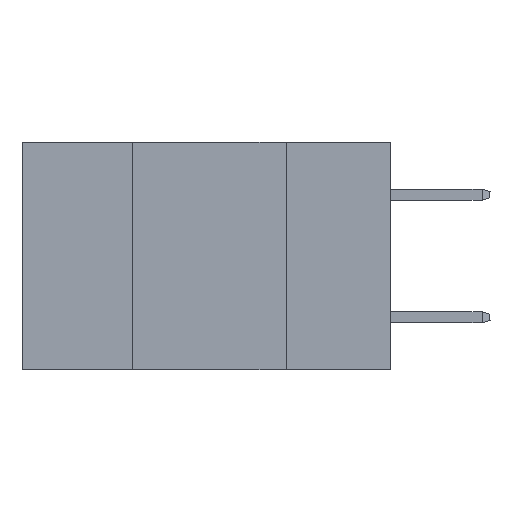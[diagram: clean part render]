
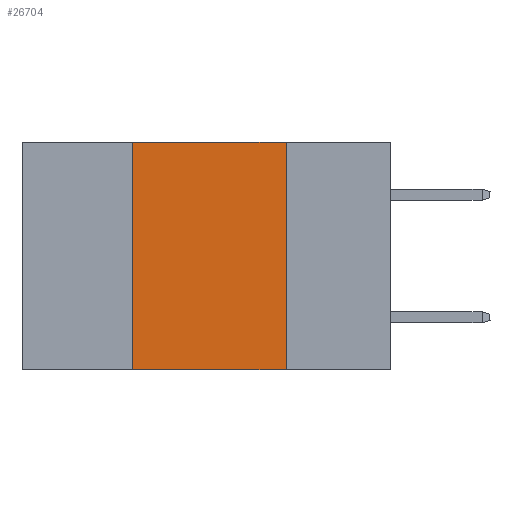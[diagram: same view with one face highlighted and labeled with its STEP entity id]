
A CAD part, left-side view. The second image highlights one B-rep face of the part: STEP entity #26704.
In plain terms, the highlighted planar face has unit normal (-1, 0, 0).
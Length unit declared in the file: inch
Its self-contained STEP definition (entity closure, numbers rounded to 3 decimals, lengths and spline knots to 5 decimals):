
#1514 = CARTESIAN_POINT ( 'NONE',  ( 0., 0.42, 0. ) ) ;
#1663 = ORIENTED_EDGE ( 'NONE', *, *, #19987, .F. ) ;
#2988 = VECTOR ( 'NONE', #11992, 39.37008 ) ;
#3080 = ORIENTED_EDGE ( 'NONE', *, *, #23069, .T. ) ;
#3209 = CARTESIAN_POINT ( 'NONE',  ( 0., 0.17, -0.37 ) ) ;
#4233 = DIRECTION ( 'NONE',  ( 0., 0., -1. ) ) ;
#6257 = VERTEX_POINT ( 'NONE', #26975 ) ;
#8599 = PLANE ( 'NONE',  #22935 ) ;
#9797 = CARTESIAN_POINT ( 'NONE',  ( 0., 0.42, 0. ) ) ;
#10349 = VERTEX_POINT ( 'NONE', #3209 ) ;
#11377 = VERTEX_POINT ( 'NONE', #1514 ) ;
#11992 = DIRECTION ( 'NONE',  ( 0., 0., 1. ) ) ;
#12355 = CARTESIAN_POINT ( 'NONE',  ( 0., 0.17, 0. ) ) ;
#12858 = EDGE_CURVE ( 'NONE', #6257, #11377, #24333, .T. ) ;
#13020 = DIRECTION ( 'NONE',  ( 1., 0., 0. ) ) ;
#14494 = LINE ( 'NONE', #26923, #21360 ) ;
#15641 = CARTESIAN_POINT ( 'NONE',  ( 0., 0.17, 0. ) ) ;
#16056 = DIRECTION ( 'NONE',  ( 0., -1., 0. ) ) ;
#16651 = ORIENTED_EDGE ( 'NONE', *, *, #20148, .F. ) ;
#16901 = VECTOR ( 'NONE', #16056, 39.37008 ) ;
#18055 = EDGE_LOOP ( 'NONE', ( #1663, #16651, #20438, #3080 ) ) ;
#19075 = FACE_OUTER_BOUND ( 'NONE', #18055, .T. ) ;
#19083 = DIRECTION ( 'NONE',  ( 0., 0., -1. ) ) ;
#19987 = EDGE_CURVE ( 'NONE', #26263, #10349, #25138, .T. ) ;
#20148 = EDGE_CURVE ( 'NONE', #11377, #26263, #14494, .T. ) ;
#20438 = ORIENTED_EDGE ( 'NONE', *, *, #12858, .F. ) ;
#21360 = VECTOR ( 'NONE', #22994, 39.37008 ) ;
#22850 = CARTESIAN_POINT ( 'NONE',  ( 0., 0.6, -0.37 ) ) ;
#22935 = AXIS2_PLACEMENT_3D ( 'NONE', #25935, #13020, #4233 ) ;
#22994 = DIRECTION ( 'NONE',  ( 0., -1., 0. ) ) ;
#23069 = EDGE_CURVE ( 'NONE', #6257, #10349, #23403, .T. ) ;
#23403 = LINE ( 'NONE', #22850, #16901 ) ;
#23415 = VECTOR ( 'NONE', #19083, 39.37008 ) ;
#24333 = LINE ( 'NONE', #9797, #2988 ) ;
#25138 = LINE ( 'NONE', #12355, #23415 ) ;
#25935 = CARTESIAN_POINT ( 'NONE',  ( 0., 0.6, 0. ) ) ;
#26263 = VERTEX_POINT ( 'NONE', #15641 ) ;
#26704 = ADVANCED_FACE ( 'NONE', ( #19075 ), #8599, .F. ) ;
#26923 = CARTESIAN_POINT ( 'NONE',  ( 0., 0.6, 0. ) ) ;
#26975 = CARTESIAN_POINT ( 'NONE',  ( 0., 0.42, -0.37 ) ) ;
